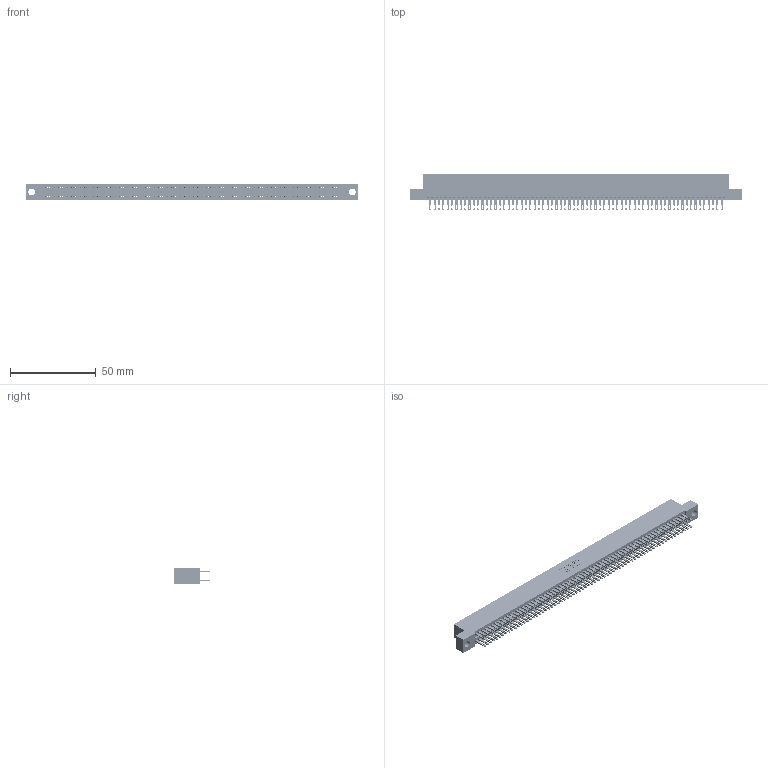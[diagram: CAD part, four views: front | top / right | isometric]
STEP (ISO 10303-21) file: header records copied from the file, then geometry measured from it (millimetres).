
FILE_DESCRIPTION (( 'STEP AP203' ), '1' );
FILE_NAME ('345-136-500-204.STEP', '2021-05-25T22:50:22', ( '' ), ( '' ), 'SwSTEP 2.0', 'SolidWorks 2020', '' );
FILE_SCHEMA (( 'CONFIG_CONTROL_DESIGN' ));
Length unit declared in the file: inch
Products named in the file (3): 345 Part_Flush Mounting Lugs - 0.156 Dia-TI; 345-136-500-204; 345-292-001_345-293-100
Assembly tree (137 placements, depth 2):
  345-136-500-204
    345 Part_Flush Mounting Lugs - 0.156 Dia-TI
    345-292-001_345-293-100  x136
Bounding box: 193.93 x 21.51 x 9.4 mm (x, y, z)
Volume: 19389.4 mm3; surface area: 30403.1 mm2
Topology: 137 solids, 137 shells, 6396 faces, 19553 edges, 13034 vertices
Faces by surface type: plane 3766, cylinder 2630
Entity records: 50203 total; most frequent: CARTESIAN_POINT 8394, ORIENTED_EDGE 8326, DIRECTION 7371, EDGE_CURVE 4163, VECTOR 3755, LINE 3755, VERTEX_POINT 2774, AXIS2_PLACEMENT_3D 1808
